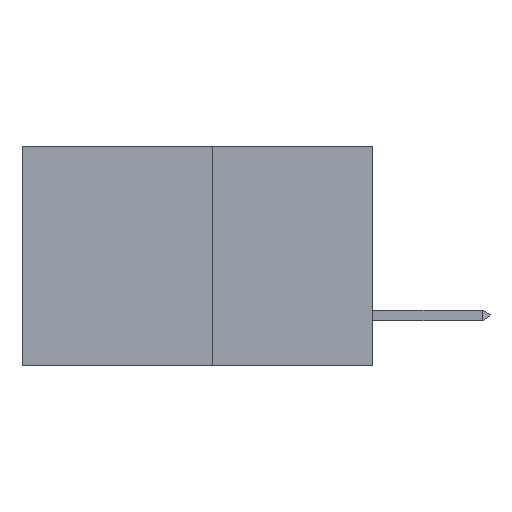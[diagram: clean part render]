
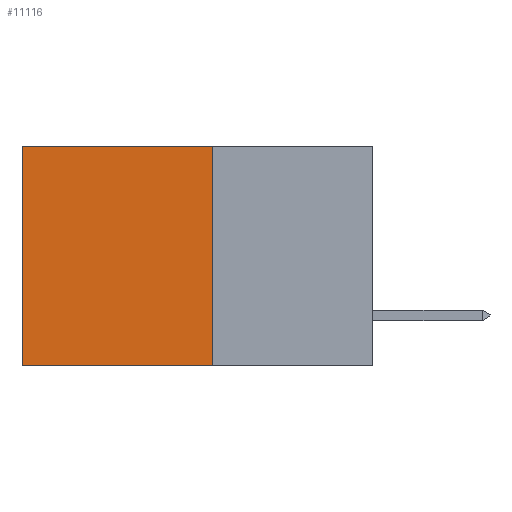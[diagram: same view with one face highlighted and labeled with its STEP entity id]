
A CAD part, left-side view. The second image highlights one B-rep face of the part: STEP entity #11116.
In plain terms, the highlighted planar face has unit normal (-1, 0, 0).
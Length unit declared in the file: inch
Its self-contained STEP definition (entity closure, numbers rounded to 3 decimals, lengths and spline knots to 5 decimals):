
#324 = DIRECTION ( 'NONE',  ( 0., 1., 0. ) ) ;
#351 = ORIENTED_EDGE ( 'NONE', *, *, #4384, .F. ) ;
#708 = EDGE_CURVE ( 'NONE', #2489, #6597, #11462, .T. ) ;
#1505 = AXIS2_PLACEMENT_3D ( 'NONE', #5570, #11700, #6443 ) ;
#1710 = VECTOR ( 'NONE', #9902, 39.37008 ) ;
#1819 = EDGE_CURVE ( 'NONE', #4589, #10036, #9849, .T. ) ;
#2218 = VECTOR ( 'NONE', #3234, 39.37008 ) ;
#2489 = VERTEX_POINT ( 'NONE', #10455 ) ;
#2491 = CARTESIAN_POINT ( 'NONE',  ( 0.277, 0.27, 0. ) ) ;
#2841 = CARTESIAN_POINT ( 'NONE',  ( 0.277, 0.27, -0.37 ) ) ;
#2878 = CARTESIAN_POINT ( 'NONE',  ( 0.277, 0.27, -0.37 ) ) ;
#2922 = VECTOR ( 'NONE', #324, 39.37008 ) ;
#3234 = DIRECTION ( 'NONE',  ( 0., 1., 0. ) ) ;
#3319 = LINE ( 'NONE', #4450, #9941 ) ;
#4101 = CARTESIAN_POINT ( 'NONE',  ( 0.277, 0.27, 0. ) ) ;
#4384 = EDGE_CURVE ( 'NONE', #4589, #2489, #11524, .T. ) ;
#4450 = CARTESIAN_POINT ( 'NONE',  ( 0.277, 0.59, -0.37 ) ) ;
#4589 = VERTEX_POINT ( 'NONE', #2491 ) ;
#4875 = CARTESIAN_POINT ( 'NONE',  ( 0.277, 0.59, -0.37 ) ) ;
#5042 = ORIENTED_EDGE ( 'NONE', *, *, #8499, .T. ) ;
#5570 = CARTESIAN_POINT ( 'NONE',  ( 0.277, 0.27, -0.37 ) ) ;
#5799 = ORIENTED_EDGE ( 'NONE', *, *, #708, .F. ) ;
#6443 = DIRECTION ( 'NONE',  ( 0., 0., -1. ) ) ;
#6597 = VERTEX_POINT ( 'NONE', #4875 ) ;
#8053 = FACE_OUTER_BOUND ( 'NONE', #11041, .T. ) ;
#8499 = EDGE_CURVE ( 'NONE', #10036, #6597, #3319, .T. ) ;
#8837 = ORIENTED_EDGE ( 'NONE', *, *, #1819, .T. ) ;
#9099 = PLANE ( 'NONE',  #1505 ) ;
#9849 = LINE ( 'NONE', #4101, #2922 ) ;
#9902 = DIRECTION ( 'NONE',  ( 0., 0., -1. ) ) ;
#9941 = VECTOR ( 'NONE', #11528, 39.37008 ) ;
#10036 = VERTEX_POINT ( 'NONE', #10243 ) ;
#10243 = CARTESIAN_POINT ( 'NONE',  ( 0.277, 0.59, 0. ) ) ;
#10455 = CARTESIAN_POINT ( 'NONE',  ( 0.277, 0.27, -0.37 ) ) ;
#11041 = EDGE_LOOP ( 'NONE', ( #5042, #5799, #351, #8837 ) ) ;
#11116 = ADVANCED_FACE ( 'NONE', ( #8053 ), #9099, .F. ) ;
#11462 = LINE ( 'NONE', #2878, #2218 ) ;
#11524 = LINE ( 'NONE', #2841, #1710 ) ;
#11528 = DIRECTION ( 'NONE',  ( 0., 0., -1. ) ) ;
#11700 = DIRECTION ( 'NONE',  ( 1., 0., 0. ) ) ;
